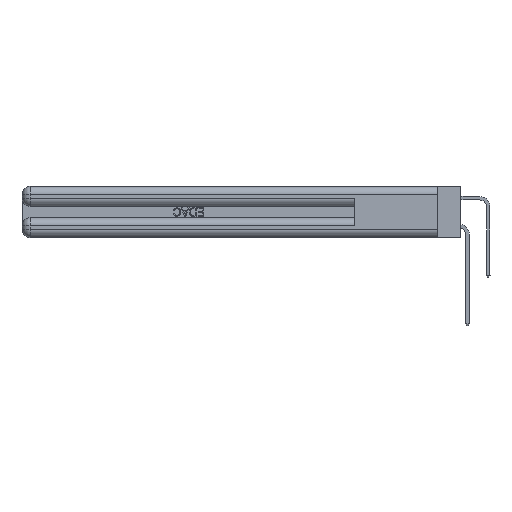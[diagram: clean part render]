
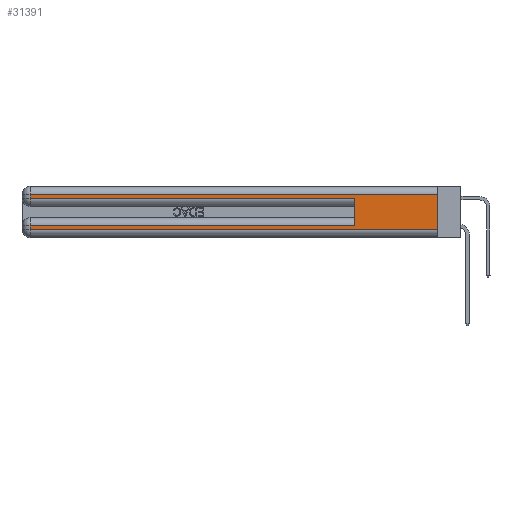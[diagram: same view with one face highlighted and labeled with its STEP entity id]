
A CAD part, left-side view. The second image highlights one B-rep face of the part: STEP entity #31391.
In plain terms, the highlighted planar face has unit normal (-1, 0, 0).
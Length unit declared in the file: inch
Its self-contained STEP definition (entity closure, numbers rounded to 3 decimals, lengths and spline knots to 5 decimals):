
#786 = LINE ( 'NONE', #15966, #32095 ) ;
#4043 = LINE ( 'NONE', #35459, #10329 ) ;
#4562 = DIRECTION ( 'NONE',  ( 1., 0., 0. ) ) ;
#4886 = ORIENTED_EDGE ( 'NONE', *, *, #40804, .T. ) ;
#6868 = CARTESIAN_POINT ( 'NONE',  ( 0., 0., 0.085 ) ) ;
#8251 = FACE_OUTER_BOUND ( 'NONE', #36649, .T. ) ;
#8698 = CARTESIAN_POINT ( 'NONE',  ( 0., 2.94, 0.085 ) ) ;
#8742 = CARTESIAN_POINT ( 'NONE',  ( 0., 0.6, 0.285 ) ) ;
#8928 = CARTESIAN_POINT ( 'NONE',  ( 0., 0.6, 0.145 ) ) ;
#10180 = CARTESIAN_POINT ( 'NONE',  ( 0., 2.94, 0.285 ) ) ;
#10329 = VECTOR ( 'NONE', #38782, 39.37008 ) ;
#12402 = VECTOR ( 'NONE', #22640, 39.37008 ) ;
#12690 = ORIENTED_EDGE ( 'NONE', *, *, #31671, .F. ) ;
#13039 = CARTESIAN_POINT ( 'NONE',  ( 0., 0., 0.285 ) ) ;
#13823 = CARTESIAN_POINT ( 'NONE',  ( 0., 2.94, 0.31 ) ) ;
#14304 = ORIENTED_EDGE ( 'NONE', *, *, #34887, .T. ) ;
#14803 = DIRECTION ( 'NONE',  ( 0., -1., 0. ) ) ;
#15828 = ORIENTED_EDGE ( 'NONE', *, *, #42305, .T. ) ;
#15966 = CARTESIAN_POINT ( 'NONE',  ( 0., 2.94, 0.37 ) ) ;
#18093 = LINE ( 'NONE', #13039, #30571 ) ;
#18463 = LINE ( 'NONE', #6868, #26296 ) ;
#18608 = CARTESIAN_POINT ( 'NONE',  ( 0., 0., 0.06 ) ) ;
#19037 = EDGE_CURVE ( 'NONE', #33905, #23352, #4043, .T. ) ;
#21195 = VECTOR ( 'NONE', #14803, 39.37008 ) ;
#21511 = VERTEX_POINT ( 'NONE', #31619 ) ;
#22611 = LINE ( 'NONE', #34186, #35702 ) ;
#22640 = DIRECTION ( 'NONE',  ( 0., 0., 1. ) ) ;
#22764 = EDGE_CURVE ( 'NONE', #40176, #31985, #786, .T. ) ;
#23352 = VERTEX_POINT ( 'NONE', #25930 ) ;
#23543 = DIRECTION ( 'NONE',  ( 0., -1., 0. ) ) ;
#25930 = CARTESIAN_POINT ( 'NONE',  ( 0., 0., 0.06 ) ) ;
#25953 = CARTESIAN_POINT ( 'NONE',  ( 0., 2.94, 0.37 ) ) ;
#26296 = VECTOR ( 'NONE', #33615, 39.37008 ) ;
#27480 = DIRECTION ( 'NONE',  ( 0., 0., -1. ) ) ;
#27540 = ORIENTED_EDGE ( 'NONE', *, *, #22764, .T. ) ;
#28088 = EDGE_CURVE ( 'NONE', #21511, #37458, #18463, .T. ) ;
#28520 = VECTOR ( 'NONE', #39387, 39.37008 ) ;
#30312 = VERTEX_POINT ( 'NONE', #8742 ) ;
#30466 = CARTESIAN_POINT ( 'NONE',  ( 0., 0., 0.31 ) ) ;
#30571 = VECTOR ( 'NONE', #23543, 39.37008 ) ;
#31130 = PLANE ( 'NONE',  #41347 ) ;
#31391 = ADVANCED_FACE ( 'NONE', ( #8251 ), #31130, .F. ) ;
#31619 = CARTESIAN_POINT ( 'NONE',  ( 0., 0.6, 0.085 ) ) ;
#31671 = EDGE_CURVE ( 'NONE', #21511, #30312, #33824, .T. ) ;
#31985 = VERTEX_POINT ( 'NONE', #10180 ) ;
#32095 = VECTOR ( 'NONE', #32942, 39.37008 ) ;
#32942 = DIRECTION ( 'NONE',  ( 0., 0., -1. ) ) ;
#33615 = DIRECTION ( 'NONE',  ( 0., 1., 0. ) ) ;
#33780 = LINE ( 'NONE', #25953, #28520 ) ;
#33824 = LINE ( 'NONE', #8928, #12402 ) ;
#33905 = VERTEX_POINT ( 'NONE', #30466 ) ;
#34028 = DIRECTION ( 'NONE',  ( 0., 1., 0. ) ) ;
#34186 = CARTESIAN_POINT ( 'NONE',  ( 0., 0., 0.31 ) ) ;
#34354 = CARTESIAN_POINT ( 'NONE',  ( 0., 0., 0.37 ) ) ;
#34887 = EDGE_CURVE ( 'NONE', #37458, #39938, #33780, .T. ) ;
#35459 = CARTESIAN_POINT ( 'NONE',  ( 0., 0., 0.37 ) ) ;
#35702 = VECTOR ( 'NONE', #34028, 39.37008 ) ;
#36649 = EDGE_LOOP ( 'NONE', ( #37980, #15828, #27540, #4886, #12690, #37727, #14304, #43089 ) ) ;
#37458 = VERTEX_POINT ( 'NONE', #8698 ) ;
#37727 = ORIENTED_EDGE ( 'NONE', *, *, #28088, .T. ) ;
#37980 = ORIENTED_EDGE ( 'NONE', *, *, #19037, .F. ) ;
#38782 = DIRECTION ( 'NONE',  ( 0., 0., -1. ) ) ;
#39387 = DIRECTION ( 'NONE',  ( 0., 0., -1. ) ) ;
#39938 = VERTEX_POINT ( 'NONE', #41706 ) ;
#40176 = VERTEX_POINT ( 'NONE', #13823 ) ;
#40458 = EDGE_CURVE ( 'NONE', #39938, #23352, #42088, .T. ) ;
#40804 = EDGE_CURVE ( 'NONE', #31985, #30312, #18093, .T. ) ;
#41347 = AXIS2_PLACEMENT_3D ( 'NONE', #34354, #4562, #27480 ) ;
#41706 = CARTESIAN_POINT ( 'NONE',  ( 0., 2.94, 0.06 ) ) ;
#42088 = LINE ( 'NONE', #18608, #21195 ) ;
#42305 = EDGE_CURVE ( 'NONE', #33905, #40176, #22611, .T. ) ;
#43089 = ORIENTED_EDGE ( 'NONE', *, *, #40458, .T. ) ;
